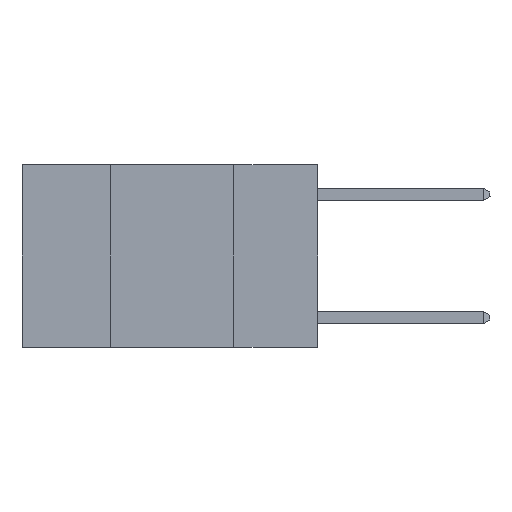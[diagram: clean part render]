
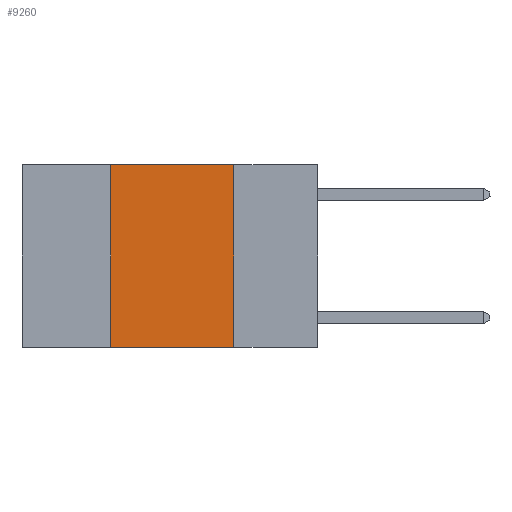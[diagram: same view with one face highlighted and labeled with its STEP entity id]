
A CAD part, left-side view. The second image highlights one B-rep face of the part: STEP entity #9260.
In plain terms, the highlighted planar face has unit normal (-1, 0, 0).
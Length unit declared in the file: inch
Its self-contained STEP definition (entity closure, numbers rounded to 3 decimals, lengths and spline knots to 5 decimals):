
#123 = LINE ( 'NONE', #10037, #8584 ) ;
#214 = ORIENTED_EDGE ( 'NONE', *, *, #4991, .F. ) ;
#265 = VERTEX_POINT ( 'NONE', #3394 ) ;
#749 = CARTESIAN_POINT ( 'NONE',  ( 0., 0.6, 0. ) ) ;
#912 = AXIS2_PLACEMENT_3D ( 'NONE', #3971, #2336, #8112 ) ;
#989 = VERTEX_POINT ( 'NONE', #1326 ) ;
#1326 = CARTESIAN_POINT ( 'NONE',  ( 0., 0.42, -0.37 ) ) ;
#1355 = DIRECTION ( 'NONE',  ( 0., -1., 0. ) ) ;
#1394 = ORIENTED_EDGE ( 'NONE', *, *, #8451, .F. ) ;
#1757 = ORIENTED_EDGE ( 'NONE', *, *, #7806, .F. ) ;
#1860 = LINE ( 'NONE', #5389, #3793 ) ;
#2110 = LINE ( 'NONE', #749, #6168 ) ;
#2336 = DIRECTION ( 'NONE',  ( 1., 0., 0. ) ) ;
#2407 = VERTEX_POINT ( 'NONE', #4048 ) ;
#2825 = EDGE_LOOP ( 'NONE', ( #1394, #214, #1757, #10306 ) ) ;
#3394 = CARTESIAN_POINT ( 'NONE',  ( 0., 0.17, -0.37 ) ) ;
#3487 = VERTEX_POINT ( 'NONE', #8422 ) ;
#3600 = CARTESIAN_POINT ( 'NONE',  ( 0., 0.17, 0. ) ) ;
#3730 = EDGE_CURVE ( 'NONE', #989, #265, #1860, .T. ) ;
#3793 = VECTOR ( 'NONE', #1355, 39.37008 ) ;
#3971 = CARTESIAN_POINT ( 'NONE',  ( 0., 0.6, 0. ) ) ;
#4016 = DIRECTION ( 'NONE',  ( 0., -1., 0. ) ) ;
#4048 = CARTESIAN_POINT ( 'NONE',  ( 0., 0.42, 0. ) ) ;
#4991 = EDGE_CURVE ( 'NONE', #2407, #3487, #2110, .T. ) ;
#5389 = CARTESIAN_POINT ( 'NONE',  ( 0., 0.6, -0.37 ) ) ;
#6000 = DIRECTION ( 'NONE',  ( 0., 0., -1. ) ) ;
#6168 = VECTOR ( 'NONE', #4016, 39.37008 ) ;
#6335 = FACE_OUTER_BOUND ( 'NONE', #2825, .T. ) ;
#6734 = VECTOR ( 'NONE', #6000, 39.37008 ) ;
#7183 = PLANE ( 'NONE',  #912 ) ;
#7698 = DIRECTION ( 'NONE',  ( 0., 0., 1. ) ) ;
#7806 = EDGE_CURVE ( 'NONE', #989, #2407, #123, .T. ) ;
#8112 = DIRECTION ( 'NONE',  ( 0., 0., -1. ) ) ;
#8422 = CARTESIAN_POINT ( 'NONE',  ( 0., 0.17, 0. ) ) ;
#8451 = EDGE_CURVE ( 'NONE', #3487, #265, #9149, .T. ) ;
#8584 = VECTOR ( 'NONE', #7698, 39.37008 ) ;
#9149 = LINE ( 'NONE', #3600, #6734 ) ;
#9260 = ADVANCED_FACE ( 'NONE', ( #6335 ), #7183, .F. ) ;
#10037 = CARTESIAN_POINT ( 'NONE',  ( 0., 0.42, 0. ) ) ;
#10306 = ORIENTED_EDGE ( 'NONE', *, *, #3730, .T. ) ;
